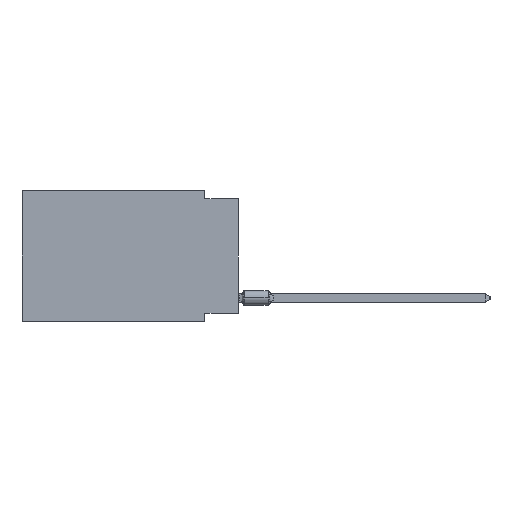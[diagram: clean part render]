
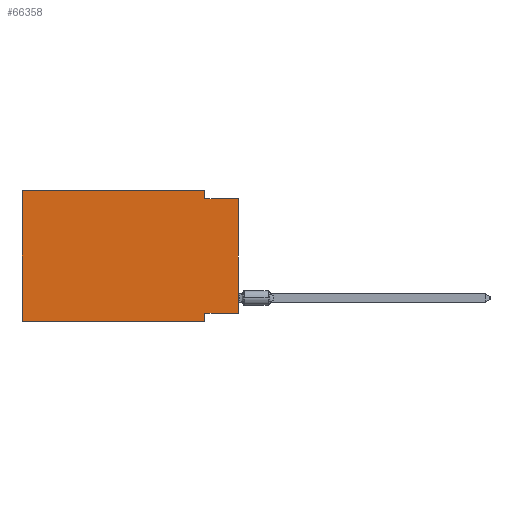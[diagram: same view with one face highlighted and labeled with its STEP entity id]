
A CAD part, left-side view. The second image highlights one B-rep face of the part: STEP entity #66358.
In plain terms, the highlighted planar face has unit normal (-1, 0, 0).
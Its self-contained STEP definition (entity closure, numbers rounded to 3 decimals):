
#320 = CARTESIAN_POINT ( 'NONE',  ( 0., 2.54, -9.906 ) ) ;
#2635 = ORIENTED_EDGE ( 'NONE', *, *, #13544, .T. ) ;
#6508 = CARTESIAN_POINT ( 'NONE',  ( 0., 0., -0.635 ) ) ;
#7141 = VECTOR ( 'NONE', #82345, 1000. ) ;
#7730 = EDGE_LOOP ( 'NONE', ( #2635, #68791, #74952, #69690, #65035, #63580, #11890, #80587 ) ) ;
#7856 = CARTESIAN_POINT ( 'NONE',  ( 0., 16.383, 0. ) ) ;
#10190 = VECTOR ( 'NONE', #75373, 1000. ) ;
#10756 = EDGE_CURVE ( 'NONE', #13923, #17274, #51212, .T. ) ;
#11052 = DIRECTION ( 'NONE',  ( 0., 0., 1. ) ) ;
#11252 = DIRECTION ( 'NONE',  ( 0., 0., -1. ) ) ;
#11890 = ORIENTED_EDGE ( 'NONE', *, *, #10756, .F. ) ;
#13544 = EDGE_CURVE ( 'NONE', #64390, #31276, #57239, .T. ) ;
#13923 = VERTEX_POINT ( 'NONE', #35182 ) ;
#15699 = DIRECTION ( 'NONE',  ( 0., 0., -1. ) ) ;
#17274 = VERTEX_POINT ( 'NONE', #320 ) ;
#19488 = EDGE_CURVE ( 'NONE', #83775, #31276, #46220, .T. ) ;
#21274 = LINE ( 'NONE', #36317, #32272 ) ;
#22119 = DIRECTION ( 'NONE',  ( 0., -1., 0. ) ) ;
#22735 = LINE ( 'NONE', #49036, #10190 ) ;
#22802 = CARTESIAN_POINT ( 'NONE',  ( 0., 0., -9.271 ) ) ;
#30477 = VECTOR ( 'NONE', #72166, 1000. ) ;
#30634 = CARTESIAN_POINT ( 'NONE',  ( 0., 0., -0.635 ) ) ;
#31276 = VERTEX_POINT ( 'NONE', #30634 ) ;
#31837 = VERTEX_POINT ( 'NONE', #57721 ) ;
#32272 = VECTOR ( 'NONE', #22119, 1000. ) ;
#32492 = VECTOR ( 'NONE', #11252, 1000. ) ;
#33428 = DIRECTION ( 'NONE',  ( 1., 0., 0. ) ) ;
#33702 = DIRECTION ( 'NONE',  ( 0., -1., 0. ) ) ;
#35182 = CARTESIAN_POINT ( 'NONE',  ( 0., 2.54, -9.271 ) ) ;
#35254 = VECTOR ( 'NONE', #77116, 1000. ) ;
#36317 = CARTESIAN_POINT ( 'NONE',  ( 0., 16.383, -9.906 ) ) ;
#36951 = CARTESIAN_POINT ( 'NONE',  ( 0., 0., 0. ) ) ;
#36975 = CARTESIAN_POINT ( 'NONE',  ( 0., 2.54, -9.906 ) ) ;
#38113 = CARTESIAN_POINT ( 'NONE',  ( 0., 16.383, -9.906 ) ) ;
#40743 = CARTESIAN_POINT ( 'NONE',  ( 0., 16.383, 0. ) ) ;
#46220 = LINE ( 'NONE', #6508, #69494 ) ;
#49036 = CARTESIAN_POINT ( 'NONE',  ( 0., 16.383, 0. ) ) ;
#51212 = LINE ( 'NONE', #36975, #35254 ) ;
#54848 = AXIS2_PLACEMENT_3D ( 'NONE', #40743, #33428, #15699 ) ;
#55598 = LINE ( 'NONE', #22802, #7141 ) ;
#57239 = LINE ( 'NONE', #36951, #67368 ) ;
#57435 = LINE ( 'NONE', #63484, #32492 ) ;
#57721 = CARTESIAN_POINT ( 'NONE',  ( 0., 2.54, 0. ) ) ;
#59759 = FACE_OUTER_BOUND ( 'NONE', #7730, .T. ) ;
#60371 = VERTEX_POINT ( 'NONE', #38113 ) ;
#61471 = EDGE_CURVE ( 'NONE', #60371, #68696, #22735, .T. ) ;
#63484 = CARTESIAN_POINT ( 'NONE',  ( 0., 2.54, 0. ) ) ;
#63580 = ORIENTED_EDGE ( 'NONE', *, *, #77160, .T. ) ;
#64390 = VERTEX_POINT ( 'NONE', #81073 ) ;
#65035 = ORIENTED_EDGE ( 'NONE', *, *, #61471, .F. ) ;
#66358 = ADVANCED_FACE ( 'NONE', ( #59759 ), #74413, .F. ) ;
#67368 = VECTOR ( 'NONE', #11052, 1000. ) ;
#67410 = CARTESIAN_POINT ( 'NONE',  ( 0., 16.383, 0. ) ) ;
#68696 = VERTEX_POINT ( 'NONE', #7856 ) ;
#68791 = ORIENTED_EDGE ( 'NONE', *, *, #19488, .F. ) ;
#69494 = VECTOR ( 'NONE', #33702, 1000. ) ;
#69690 = ORIENTED_EDGE ( 'NONE', *, *, #72359, .F. ) ;
#72166 = DIRECTION ( 'NONE',  ( 0., -1., 0. ) ) ;
#72359 = EDGE_CURVE ( 'NONE', #68696, #31837, #73458, .T. ) ;
#72979 = EDGE_CURVE ( 'NONE', #64390, #13923, #55598, .T. ) ;
#73458 = LINE ( 'NONE', #67410, #30477 ) ;
#74413 = PLANE ( 'NONE',  #54848 ) ;
#74952 = ORIENTED_EDGE ( 'NONE', *, *, #76107, .F. ) ;
#75373 = DIRECTION ( 'NONE',  ( 0., 0., 1. ) ) ;
#76107 = EDGE_CURVE ( 'NONE', #31837, #83775, #57435, .T. ) ;
#77116 = DIRECTION ( 'NONE',  ( 0., 0., -1. ) ) ;
#77160 = EDGE_CURVE ( 'NONE', #60371, #17274, #21274, .T. ) ;
#79036 = CARTESIAN_POINT ( 'NONE',  ( 0., 2.54, -0.635 ) ) ;
#80587 = ORIENTED_EDGE ( 'NONE', *, *, #72979, .F. ) ;
#81073 = CARTESIAN_POINT ( 'NONE',  ( 0., 0., -9.271 ) ) ;
#82345 = DIRECTION ( 'NONE',  ( 0., 1., 0. ) ) ;
#83775 = VERTEX_POINT ( 'NONE', #79036 ) ;
